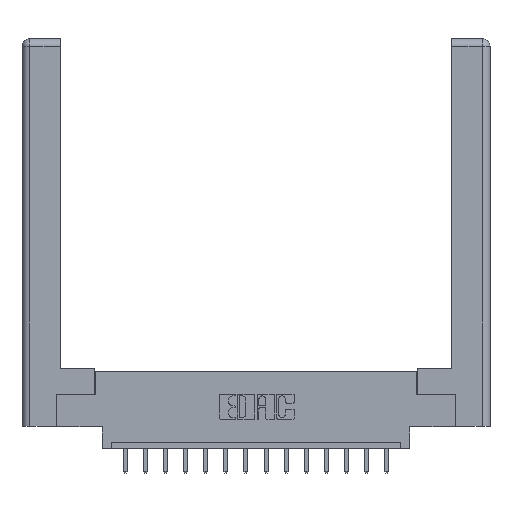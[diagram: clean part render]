
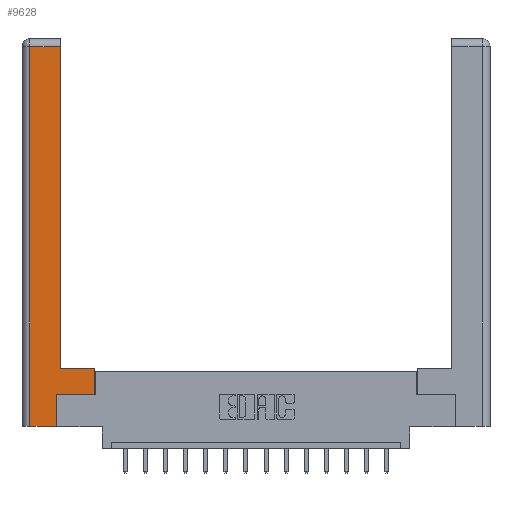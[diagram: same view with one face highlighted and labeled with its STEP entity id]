
A CAD part, top view. The second image highlights one B-rep face of the part: STEP entity #9628.
In plain terms, the highlighted planar face has unit normal (0, 0, 1).
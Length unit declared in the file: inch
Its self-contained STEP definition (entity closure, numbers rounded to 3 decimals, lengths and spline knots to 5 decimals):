
#179 = EDGE_CURVE ( 'NONE', #3536, #10947, #2252, .T. ) ;
#273 = VERTEX_POINT ( 'NONE', #11809 ) ;
#403 = LINE ( 'NONE', #10864, #14837 ) ;
#1087 = CARTESIAN_POINT ( 'NONE',  ( 0.295, 0.45, 0. ) ) ;
#1102 = EDGE_CURVE ( 'NONE', #10947, #3411, #14662, .T. ) ;
#1429 = DIRECTION ( 'NONE',  ( 0., 0., -1. ) ) ;
#1505 = LINE ( 'NONE', #13187, #10287 ) ;
#1515 = VERTEX_POINT ( 'NONE', #9165 ) ;
#2001 = ORIENTED_EDGE ( 'NONE', *, *, #9962, .T. ) ;
#2042 = CARTESIAN_POINT ( 'NONE',  ( 0.265, 0.245, 0. ) ) ;
#2252 = LINE ( 'NONE', #6673, #15720 ) ;
#2275 = ORIENTED_EDGE ( 'NONE', *, *, #7956, .T. ) ;
#2422 = PLANE ( 'NONE',  #3191 ) ;
#2446 = LINE ( 'NONE', #1087, #5959 ) ;
#2899 = DIRECTION ( 'NONE',  ( 0., 1., 0. ) ) ;
#3191 = AXIS2_PLACEMENT_3D ( 'NONE', #6661, #1429, #5300 ) ;
#3411 = VERTEX_POINT ( 'NONE', #14203 ) ;
#3536 = VERTEX_POINT ( 'NONE', #9255 ) ;
#3642 = DIRECTION ( 'NONE',  ( -1., 0., 0. ) ) ;
#3858 = CARTESIAN_POINT ( 'NONE',  ( 0.265, 0., 0. ) ) ;
#3970 = VECTOR ( 'NONE', #2899, 39.37008 ) ;
#4215 = CARTESIAN_POINT ( 'NONE',  ( 0.0615, 0., 0. ) ) ;
#5300 = DIRECTION ( 'NONE',  ( -1., 0., 0. ) ) ;
#5353 = VERTEX_POINT ( 'NONE', #15418 ) ;
#5387 = EDGE_CURVE ( 'NONE', #273, #5353, #1505, .T. ) ;
#5837 = DIRECTION ( 'NONE',  ( 0., 1., 0. ) ) ;
#5935 = DIRECTION ( 'NONE',  ( 0., 1., 0. ) ) ;
#5959 = VECTOR ( 'NONE', #3642, 39.37008 ) ;
#6661 = CARTESIAN_POINT ( 'NONE',  ( 0., 0., 0. ) ) ;
#6673 = CARTESIAN_POINT ( 'NONE',  ( 0.265, 0., 0. ) ) ;
#6824 = LINE ( 'NONE', #4215, #11347 ) ;
#7125 = VECTOR ( 'NONE', #5837, 39.37008 ) ;
#7378 = CARTESIAN_POINT ( 'NONE',  ( 0.295, 3., 0. ) ) ;
#7846 = ORIENTED_EDGE ( 'NONE', *, *, #9971, .T. ) ;
#7956 = EDGE_CURVE ( 'NONE', #3411, #1515, #403, .T. ) ;
#8004 = CARTESIAN_POINT ( 'NONE',  ( 0.565, 0.45, 0. ) ) ;
#9165 = CARTESIAN_POINT ( 'NONE',  ( 0.565, 0.245, 0. ) ) ;
#9255 = CARTESIAN_POINT ( 'NONE',  ( 0.0615, 0., 0. ) ) ;
#9336 = ORIENTED_EDGE ( 'NONE', *, *, #13944, .T. ) ;
#9628 = ADVANCED_FACE ( 'NONE', ( #9751 ), #2422, .F. ) ;
#9751 = FACE_OUTER_BOUND ( 'NONE', #16193, .T. ) ;
#9763 = DIRECTION ( 'NONE',  ( 1., 0., 0. ) ) ;
#9962 = EDGE_CURVE ( 'NONE', #1515, #10332, #13745, .T. ) ;
#9971 = EDGE_CURVE ( 'NONE', #5353, #3536, #6824, .T. ) ;
#10287 = VECTOR ( 'NONE', #10467, 39.37008 ) ;
#10332 = VERTEX_POINT ( 'NONE', #15783 ) ;
#10467 = DIRECTION ( 'NONE',  ( -1., 0., 0. ) ) ;
#10674 = DIRECTION ( 'NONE',  ( 0., -1., 0. ) ) ;
#10864 = CARTESIAN_POINT ( 'NONE',  ( 0.565, 0.245, 0. ) ) ;
#10947 = VERTEX_POINT ( 'NONE', #3858 ) ;
#11011 = LINE ( 'NONE', #7378, #7125 ) ;
#11347 = VECTOR ( 'NONE', #10674, 39.37008 ) ;
#11509 = VERTEX_POINT ( 'NONE', #16401 ) ;
#11767 = ORIENTED_EDGE ( 'NONE', *, *, #15362, .T. ) ;
#11809 = CARTESIAN_POINT ( 'NONE',  ( 0.295, 2.94, 0. ) ) ;
#12930 = ORIENTED_EDGE ( 'NONE', *, *, #5387, .T. ) ;
#13187 = CARTESIAN_POINT ( 'NONE',  ( 0.0615, 2.94, 0. ) ) ;
#13507 = ORIENTED_EDGE ( 'NONE', *, *, #1102, .T. ) ;
#13745 = LINE ( 'NONE', #8004, #3970 ) ;
#13944 = EDGE_CURVE ( 'NONE', #10332, #11509, #2446, .T. ) ;
#14203 = CARTESIAN_POINT ( 'NONE',  ( 0.265, 0.245, 0. ) ) ;
#14441 = DIRECTION ( 'NONE',  ( 1., 0., 0. ) ) ;
#14662 = LINE ( 'NONE', #2042, #15717 ) ;
#14837 = VECTOR ( 'NONE', #9763, 39.37008 ) ;
#15362 = EDGE_CURVE ( 'NONE', #11509, #273, #11011, .T. ) ;
#15418 = CARTESIAN_POINT ( 'NONE',  ( 0.0615, 2.94, 0. ) ) ;
#15717 = VECTOR ( 'NONE', #5935, 39.37008 ) ;
#15720 = VECTOR ( 'NONE', #14441, 39.37008 ) ;
#15762 = ORIENTED_EDGE ( 'NONE', *, *, #179, .T. ) ;
#15783 = CARTESIAN_POINT ( 'NONE',  ( 0.565, 0.45, 0. ) ) ;
#16193 = EDGE_LOOP ( 'NONE', ( #11767, #12930, #7846, #15762, #13507, #2275, #2001, #9336 ) ) ;
#16401 = CARTESIAN_POINT ( 'NONE',  ( 0.295, 0.45, 0. ) ) ;
